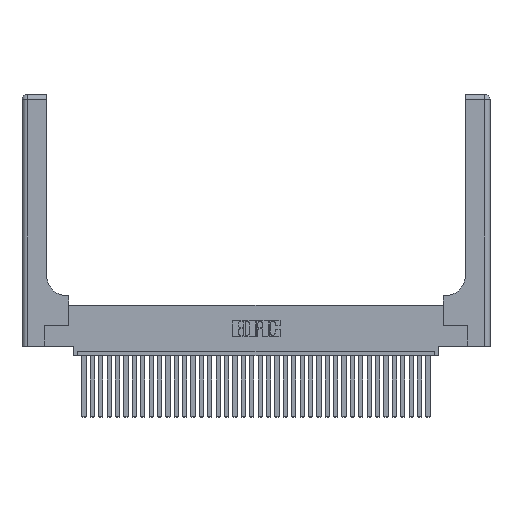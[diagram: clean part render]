
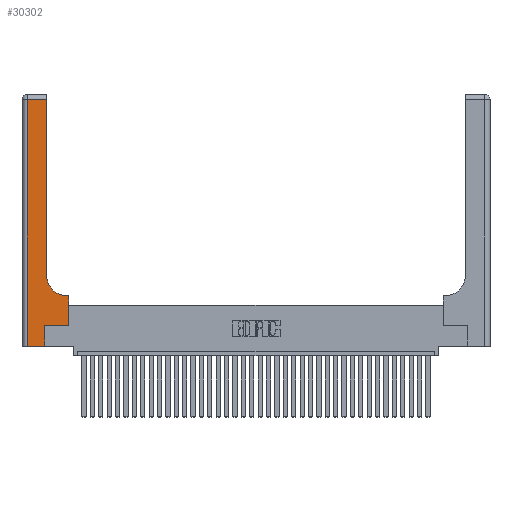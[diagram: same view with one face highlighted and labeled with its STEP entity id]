
A CAD part, top view. The second image highlights one B-rep face of the part: STEP entity #30302.
In plain terms, the highlighted planar face has unit normal (0, 0, 1).
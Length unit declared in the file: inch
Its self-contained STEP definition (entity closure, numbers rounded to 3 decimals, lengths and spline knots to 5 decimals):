
#265 = DIRECTION ( 'NONE',  ( 1., 0., 0. ) ) ;
#1064 = LINE ( 'NONE', #17745, #23723 ) ;
#1211 = CARTESIAN_POINT ( 'NONE',  ( 0., 3., 0.37 ) ) ;
#1601 = AXIS2_PLACEMENT_3D ( 'NONE', #28229, #13923, #14299 ) ;
#2037 = VERTEX_POINT ( 'NONE', #31400 ) ;
#3132 = ORIENTED_EDGE ( 'NONE', *, *, #5512, .T. ) ;
#3562 = VERTEX_POINT ( 'NONE', #8087 ) ;
#3941 = PLANE ( 'NONE',  #35342 ) ;
#4243 = EDGE_CURVE ( 'NONE', #2037, #3562, #18533, .T. ) ;
#4609 = VECTOR ( 'NONE', #7468, 39.37008 ) ;
#4640 = VERTEX_POINT ( 'NONE', #33148 ) ;
#5512 = EDGE_CURVE ( 'NONE', #27909, #36324, #25104, .T. ) ;
#5689 = DIRECTION ( 'NONE',  ( -1., 0., 0. ) ) ;
#6651 = ORIENTED_EDGE ( 'NONE', *, *, #32191, .T. ) ;
#7191 = ORIENTED_EDGE ( 'NONE', *, *, #19583, .T. ) ;
#7216 = CARTESIAN_POINT ( 'NONE',  ( 0.5415, 0.6, 0.37 ) ) ;
#7468 = DIRECTION ( 'NONE',  ( 0., -1., 0. ) ) ;
#8057 = CARTESIAN_POINT ( 'NONE',  ( 0., 2.94, 0.37 ) ) ;
#8087 = CARTESIAN_POINT ( 'NONE',  ( 0.06, 2.94, 0.37 ) ) ;
#8628 = EDGE_CURVE ( 'NONE', #12951, #27909, #30095, .T. ) ;
#9108 = EDGE_LOOP ( 'NONE', ( #34076, #18117, #6651, #7191, #17880, #28474, #34441, #3132, #20232 ) ) ;
#9425 = VECTOR ( 'NONE', #31590, 39.37008 ) ;
#9916 = CARTESIAN_POINT ( 'NONE',  ( 0.269, 0., 0.37 ) ) ;
#11102 = VERTEX_POINT ( 'NONE', #24634 ) ;
#11131 = EDGE_CURVE ( 'NONE', #30645, #12951, #20080, .T. ) ;
#11496 = CARTESIAN_POINT ( 'NONE',  ( 0.269, 0.25, 0.37 ) ) ;
#12227 = CARTESIAN_POINT ( 'NONE',  ( 0.2915, 3., 0.37 ) ) ;
#12951 = VERTEX_POINT ( 'NONE', #18708 ) ;
#13143 = DIRECTION ( 'NONE',  ( 0., 1., 0. ) ) ;
#13919 = LINE ( 'NONE', #24602, #4609 ) ;
#13923 = DIRECTION ( 'NONE',  ( 0., 0., -1. ) ) ;
#14299 = DIRECTION ( 'NONE',  ( 1., 0., 0. ) ) ;
#15189 = DIRECTION ( 'NONE',  ( -1., 0., 0. ) ) ;
#17745 = CARTESIAN_POINT ( 'NONE',  ( 0., 0., 0.37 ) ) ;
#17880 = ORIENTED_EDGE ( 'NONE', *, *, #25316, .T. ) ;
#18117 = ORIENTED_EDGE ( 'NONE', *, *, #4243, .T. ) ;
#18533 = LINE ( 'NONE', #8057, #27900 ) ;
#18708 = CARTESIAN_POINT ( 'NONE',  ( 0.5585, 0.25, 0.37 ) ) ;
#18831 = DIRECTION ( 'NONE',  ( -1., 0., 0. ) ) ;
#19347 = EDGE_CURVE ( 'NONE', #36324, #35665, #25076, .T. ) ;
#19583 = EDGE_CURVE ( 'NONE', #4640, #11102, #1064, .T. ) ;
#19894 = FACE_OUTER_BOUND ( 'NONE', #9108, .T. ) ;
#20080 = LINE ( 'NONE', #25275, #9425 ) ;
#20145 = CARTESIAN_POINT ( 'NONE',  ( 0.5585, 0.25, 0.37 ) ) ;
#20232 = ORIENTED_EDGE ( 'NONE', *, *, #19347, .T. ) ;
#20748 = EDGE_CURVE ( 'NONE', #35665, #2037, #32955, .T. ) ;
#22943 = LINE ( 'NONE', #9916, #31831 ) ;
#23723 = VECTOR ( 'NONE', #265, 39.37008 ) ;
#23848 = VECTOR ( 'NONE', #13143, 39.37008 ) ;
#24051 = DIRECTION ( 'NONE',  ( 0., 0., -1. ) ) ;
#24602 = CARTESIAN_POINT ( 'NONE',  ( 0.06, 3., 0.37 ) ) ;
#24634 = CARTESIAN_POINT ( 'NONE',  ( 0.269, 0., 0.37 ) ) ;
#25071 = CARTESIAN_POINT ( 'NONE',  ( 0.5585, 0.6, 0.37 ) ) ;
#25076 = CIRCLE ( 'NONE', #1601, 0.25 ) ;
#25104 = LINE ( 'NONE', #34425, #27316 ) ;
#25275 = CARTESIAN_POINT ( 'NONE',  ( 0.269, 0.25, 0.37 ) ) ;
#25316 = EDGE_CURVE ( 'NONE', #11102, #30645, #22943, .T. ) ;
#26683 = DIRECTION ( 'NONE',  ( 0., 1., 0. ) ) ;
#27316 = VECTOR ( 'NONE', #5689, 39.37008 ) ;
#27900 = VECTOR ( 'NONE', #18831, 39.37008 ) ;
#27909 = VERTEX_POINT ( 'NONE', #25071 ) ;
#28229 = CARTESIAN_POINT ( 'NONE',  ( 0.5415, 0.85, 0.37 ) ) ;
#28474 = ORIENTED_EDGE ( 'NONE', *, *, #11131, .T. ) ;
#28999 = DIRECTION ( 'NONE',  ( 0., 1., 0. ) ) ;
#30095 = LINE ( 'NONE', #20145, #23848 ) ;
#30302 = ADVANCED_FACE ( 'NONE', ( #19894 ), #3941, .F. ) ;
#30645 = VERTEX_POINT ( 'NONE', #11496 ) ;
#31400 = CARTESIAN_POINT ( 'NONE',  ( 0.2915, 2.94, 0.37 ) ) ;
#31590 = DIRECTION ( 'NONE',  ( 1., 0., 0. ) ) ;
#31831 = VECTOR ( 'NONE', #26683, 39.37008 ) ;
#32117 = CARTESIAN_POINT ( 'NONE',  ( 0.2915, 0.85, 0.37 ) ) ;
#32191 = EDGE_CURVE ( 'NONE', #3562, #4640, #13919, .T. ) ;
#32955 = LINE ( 'NONE', #12227, #33835 ) ;
#33148 = CARTESIAN_POINT ( 'NONE',  ( 0.06, 0., 0.37 ) ) ;
#33835 = VECTOR ( 'NONE', #28999, 39.37008 ) ;
#34076 = ORIENTED_EDGE ( 'NONE', *, *, #20748, .T. ) ;
#34425 = CARTESIAN_POINT ( 'NONE',  ( 0.2915, 0.6, 0.37 ) ) ;
#34441 = ORIENTED_EDGE ( 'NONE', *, *, #8628, .T. ) ;
#35342 = AXIS2_PLACEMENT_3D ( 'NONE', #1211, #24051, #15189 ) ;
#35665 = VERTEX_POINT ( 'NONE', #32117 ) ;
#36324 = VERTEX_POINT ( 'NONE', #7216 ) ;
